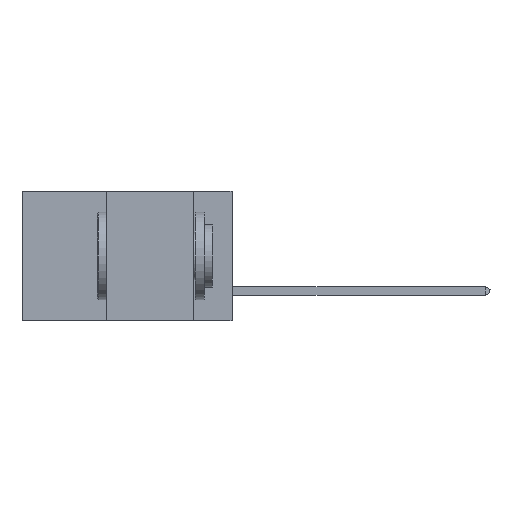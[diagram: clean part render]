
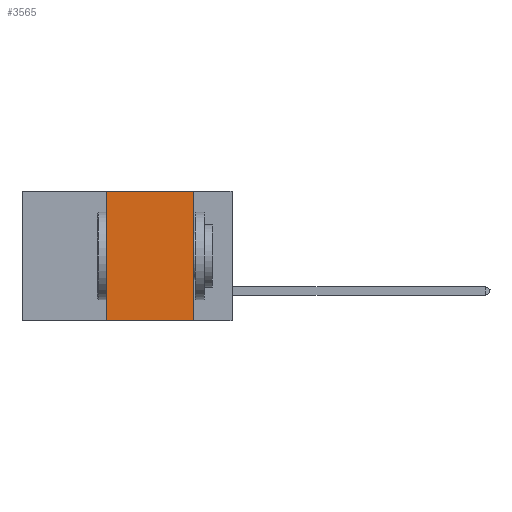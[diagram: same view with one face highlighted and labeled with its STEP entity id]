
A CAD part, left-side view. The second image highlights one B-rep face of the part: STEP entity #3565.
In plain terms, the highlighted planar face has unit normal (-1, 0, 0).
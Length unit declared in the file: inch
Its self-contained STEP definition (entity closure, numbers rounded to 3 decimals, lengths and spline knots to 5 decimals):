
#58 = ORIENTED_EDGE ( 'NONE', *, *, #11481, .F. ) ;
#475 = VERTEX_POINT ( 'NONE', #7114 ) ;
#1330 = CARTESIAN_POINT ( 'NONE',  ( 0., 0.11, 0. ) ) ;
#1942 = CARTESIAN_POINT ( 'NONE',  ( 0., 0.6, -0.37 ) ) ;
#2052 = VERTEX_POINT ( 'NONE', #4147 ) ;
#2310 = EDGE_CURVE ( 'NONE', #2052, #8888, #5381, .T. ) ;
#3019 = VECTOR ( 'NONE', #12288, 39.37008 ) ;
#3230 = CARTESIAN_POINT ( 'NONE',  ( 0., 0.11, -0.37 ) ) ;
#3565 = ADVANCED_FACE ( 'NONE', ( #6742 ), #7730, .F. ) ;
#4117 = EDGE_CURVE ( 'NONE', #475, #8888, #5337, .T. ) ;
#4147 = CARTESIAN_POINT ( 'NONE',  ( 0., 0.36, -0.37 ) ) ;
#5337 = LINE ( 'NONE', #1330, #5948 ) ;
#5381 = LINE ( 'NONE', #1942, #12548 ) ;
#5926 = ORIENTED_EDGE ( 'NONE', *, *, #4117, .F. ) ;
#5944 = LINE ( 'NONE', #8555, #3019 ) ;
#5948 = VECTOR ( 'NONE', #11976, 39.37008 ) ;
#6572 = CARTESIAN_POINT ( 'NONE',  ( 0., 0.36, 0. ) ) ;
#6596 = EDGE_CURVE ( 'NONE', #8361, #475, #11403, .T. ) ;
#6624 = CARTESIAN_POINT ( 'NONE',  ( 0., 0.6, 0. ) ) ;
#6742 = FACE_OUTER_BOUND ( 'NONE', #12619, .T. ) ;
#7114 = CARTESIAN_POINT ( 'NONE',  ( 0., 0.11, 0. ) ) ;
#7730 = PLANE ( 'NONE',  #11639 ) ;
#8361 = VERTEX_POINT ( 'NONE', #6572 ) ;
#8555 = CARTESIAN_POINT ( 'NONE',  ( 0., 0.36, 0. ) ) ;
#8798 = DIRECTION ( 'NONE',  ( 0., -1., 0. ) ) ;
#8800 = VECTOR ( 'NONE', #11904, 39.37008 ) ;
#8888 = VERTEX_POINT ( 'NONE', #3230 ) ;
#10298 = ORIENTED_EDGE ( 'NONE', *, *, #6596, .F. ) ;
#10606 = DIRECTION ( 'NONE',  ( 0., 0., -1. ) ) ;
#11403 = LINE ( 'NONE', #12276, #8800 ) ;
#11481 = EDGE_CURVE ( 'NONE', #2052, #8361, #5944, .T. ) ;
#11639 = AXIS2_PLACEMENT_3D ( 'NONE', #6624, #12556, #10606 ) ;
#11904 = DIRECTION ( 'NONE',  ( 0., -1., 0. ) ) ;
#11976 = DIRECTION ( 'NONE',  ( 0., 0., -1. ) ) ;
#12276 = CARTESIAN_POINT ( 'NONE',  ( 0., 0.6, 0. ) ) ;
#12288 = DIRECTION ( 'NONE',  ( 0., 0., 1. ) ) ;
#12311 = ORIENTED_EDGE ( 'NONE', *, *, #2310, .T. ) ;
#12548 = VECTOR ( 'NONE', #8798, 39.37008 ) ;
#12556 = DIRECTION ( 'NONE',  ( 1., 0., 0. ) ) ;
#12619 = EDGE_LOOP ( 'NONE', ( #5926, #10298, #58, #12311 ) ) ;
